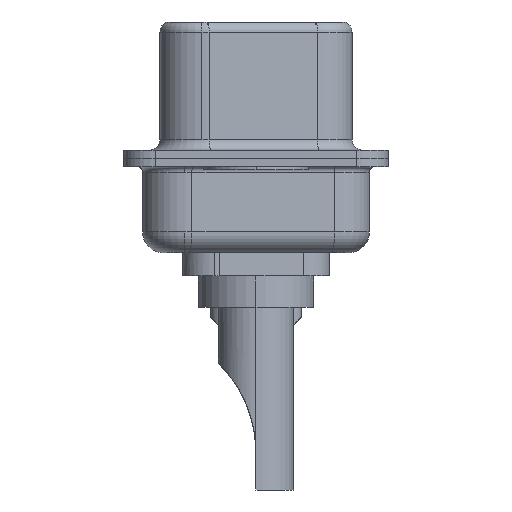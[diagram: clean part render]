
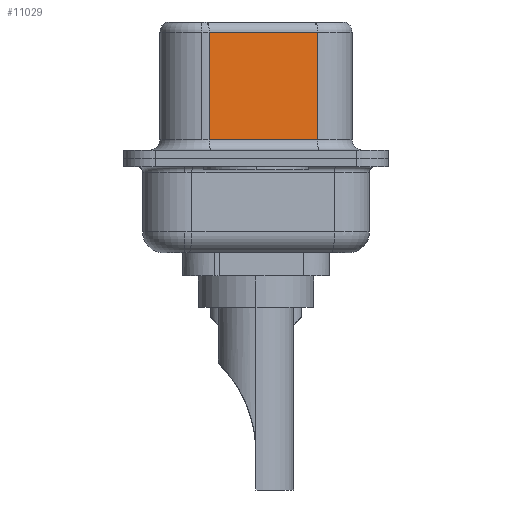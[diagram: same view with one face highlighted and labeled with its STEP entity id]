
A CAD part, left-side view. The second image highlights one B-rep face of the part: STEP entity #11029.
In plain terms, the highlighted planar face has unit normal (-0.985, -0.174, 0).
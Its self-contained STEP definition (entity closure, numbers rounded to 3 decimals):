
#358 = VECTOR ( 'NONE', #20408, 1000. ) ;
#1098 = ORIENTED_EDGE ( 'NONE', *, *, #12264, .T. ) ;
#1212 = FACE_OUTER_BOUND ( 'NONE', #2081, .T. ) ;
#1684 = CARTESIAN_POINT ( 'NONE',  ( 4.58, -2.927, 6.52 ) ) ;
#1976 = CARTESIAN_POINT ( 'NONE',  ( 3.67, 2.233, 0.9 ) ) ;
#2081 = EDGE_LOOP ( 'NONE', ( #3794, #6961, #8222, #1098 ) ) ;
#2920 = CARTESIAN_POINT ( 'NONE',  ( 3.67, 2.233, 6.02 ) ) ;
#3229 = VECTOR ( 'NONE', #5303, 1000. ) ;
#3794 = ORIENTED_EDGE ( 'NONE', *, *, #18583, .F. ) ;
#4284 = VERTEX_POINT ( 'NONE', #13935 ) ;
#5303 = DIRECTION ( 'NONE',  ( 0.174, -0.985, 0. ) ) ;
#5504 = EDGE_CURVE ( 'NONE', #10259, #8018, #13601, .T. ) ;
#5773 = CARTESIAN_POINT ( 'NONE',  ( 4.58, -2.927, 6.02 ) ) ;
#6961 = ORIENTED_EDGE ( 'NONE', *, *, #16820, .T. ) ;
#8018 = VERTEX_POINT ( 'NONE', #1976 ) ;
#8222 = ORIENTED_EDGE ( 'NONE', *, *, #5504, .T. ) ;
#8343 = PLANE ( 'NONE',  #15273 ) ;
#8822 = VERTEX_POINT ( 'NONE', #15869 ) ;
#9258 = DIRECTION ( 'NONE',  ( 0., 0., -1. ) ) ;
#9549 = LINE ( 'NONE', #5773, #358 ) ;
#9960 = DIRECTION ( 'NONE',  ( -0.174, 0.985, 0. ) ) ;
#10259 = VERTEX_POINT ( 'NONE', #2920 ) ;
#11029 = ADVANCED_FACE ( 'NONE', ( #1212 ), #8343, .F. ) ;
#11409 = LINE ( 'NONE', #15039, #3229 ) ;
#12264 = EDGE_CURVE ( 'NONE', #8018, #8822, #11409, .T. ) ;
#12542 = LINE ( 'NONE', #15593, #17370 ) ;
#13601 = LINE ( 'NONE', #13833, #17899 ) ;
#13833 = CARTESIAN_POINT ( 'NONE',  ( 3.67, 2.233, 6.52 ) ) ;
#13935 = CARTESIAN_POINT ( 'NONE',  ( 4.58, -2.927, 6.02 ) ) ;
#15039 = CARTESIAN_POINT ( 'NONE',  ( 4.58, -2.927, 0.9 ) ) ;
#15273 = AXIS2_PLACEMENT_3D ( 'NONE', #1684, #19695, #9960 ) ;
#15593 = CARTESIAN_POINT ( 'NONE',  ( 4.58, -2.927, 6.52 ) ) ;
#15869 = CARTESIAN_POINT ( 'NONE',  ( 4.58, -2.927, 0.9 ) ) ;
#16820 = EDGE_CURVE ( 'NONE', #4284, #10259, #9549, .T. ) ;
#17370 = VECTOR ( 'NONE', #20439, 1000. ) ;
#17899 = VECTOR ( 'NONE', #9258, 1000. ) ;
#18583 = EDGE_CURVE ( 'NONE', #4284, #8822, #12542, .T. ) ;
#19695 = DIRECTION ( 'NONE',  ( 0.985, 0.174, 0. ) ) ;
#20408 = DIRECTION ( 'NONE',  ( -0.174, 0.985, 0. ) ) ;
#20439 = DIRECTION ( 'NONE',  ( 0., 0., -1. ) ) ;
